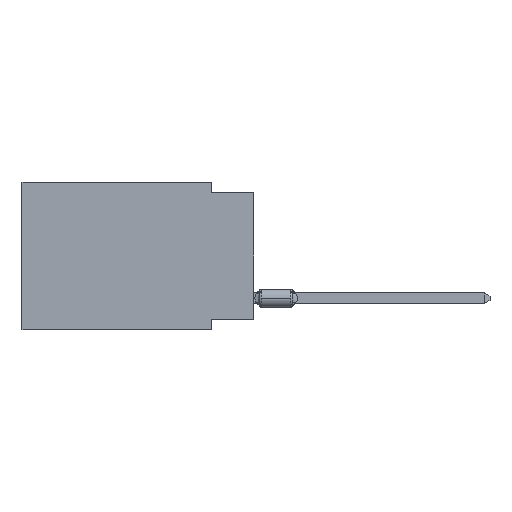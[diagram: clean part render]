
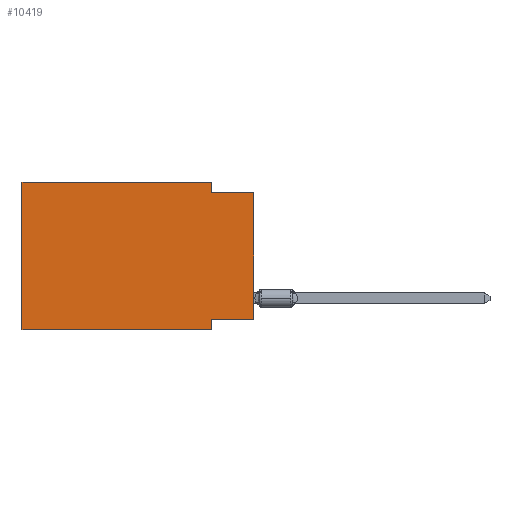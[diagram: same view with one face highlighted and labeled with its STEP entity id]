
A CAD part, left-side view. The second image highlights one B-rep face of the part: STEP entity #10419.
In plain terms, the highlighted planar face has unit normal (-1, 0, 0).
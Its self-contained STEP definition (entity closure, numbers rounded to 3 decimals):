
#98 = LINE ( 'NONE', #17383, #18273 ) ;
#118 = CARTESIAN_POINT ( 'NONE',  ( 0., 13.97, 0. ) ) ;
#355 = ORIENTED_EDGE ( 'NONE', *, *, #24967, .F. ) ;
#818 = EDGE_CURVE ( 'NONE', #24114, #4047, #17471, .T. ) ;
#2489 = DIRECTION ( 'NONE',  ( 0., 0., 1. ) ) ;
#2927 = LINE ( 'NONE', #19809, #13702 ) ;
#2941 = CARTESIAN_POINT ( 'NONE',  ( 0., 0., -8.255 ) ) ;
#3086 = DIRECTION ( 'NONE',  ( 0., -1., 0. ) ) ;
#3266 = AXIS2_PLACEMENT_3D ( 'NONE', #118, #14785, #27245 ) ;
#4047 = VERTEX_POINT ( 'NONE', #27124 ) ;
#4933 = EDGE_CURVE ( 'NONE', #27337, #19871, #8294, .T. ) ;
#5294 = CARTESIAN_POINT ( 'NONE',  ( 0., 13.97, -8.89 ) ) ;
#5333 = EDGE_CURVE ( 'NONE', #19871, #11770, #98, .T. ) ;
#5470 = VECTOR ( 'NONE', #3086, 1000. ) ;
#6380 = CARTESIAN_POINT ( 'NONE',  ( 0., 2.54, 0. ) ) ;
#6936 = CARTESIAN_POINT ( 'NONE',  ( 0., 0., -8.255 ) ) ;
#7113 = EDGE_CURVE ( 'NONE', #27337, #24316, #22320, .T. ) ;
#8066 = LINE ( 'NONE', #21229, #18975 ) ;
#8294 = LINE ( 'NONE', #16730, #24438 ) ;
#8352 = DIRECTION ( 'NONE',  ( 0., 0., 1. ) ) ;
#10286 = CARTESIAN_POINT ( 'NONE',  ( 0., 0., 0. ) ) ;
#10288 = VERTEX_POINT ( 'NONE', #22146 ) ;
#10419 = ADVANCED_FACE ( 'NONE', ( #19072 ), #16859, .F. ) ;
#10616 = ORIENTED_EDGE ( 'NONE', *, *, #5333, .F. ) ;
#10738 = ORIENTED_EDGE ( 'NONE', *, *, #4933, .F. ) ;
#11770 = VERTEX_POINT ( 'NONE', #6380 ) ;
#11837 = DIRECTION ( 'NONE',  ( 0., 0., -1. ) ) ;
#12304 = VECTOR ( 'NONE', #8352, 1000. ) ;
#12635 = LINE ( 'NONE', #10286, #12304 ) ;
#13702 = VECTOR ( 'NONE', #17733, 1000. ) ;
#13925 = CARTESIAN_POINT ( 'NONE',  ( 0., 2.54, 0. ) ) ;
#14785 = DIRECTION ( 'NONE',  ( 1., 0., 0. ) ) ;
#15174 = VERTEX_POINT ( 'NONE', #18617 ) ;
#15389 = DIRECTION ( 'NONE',  ( 0., 1., 0. ) ) ;
#15802 = VECTOR ( 'NONE', #15389, 1000. ) ;
#16543 = CARTESIAN_POINT ( 'NONE',  ( 0., 13.97, 0. ) ) ;
#16730 = CARTESIAN_POINT ( 'NONE',  ( 0., 13.97, 0. ) ) ;
#16859 = PLANE ( 'NONE',  #3266 ) ;
#17247 = ORIENTED_EDGE ( 'NONE', *, *, #27040, .T. ) ;
#17248 = DIRECTION ( 'NONE',  ( 0., -1., 0. ) ) ;
#17383 = CARTESIAN_POINT ( 'NONE',  ( 0., 13.97, 0. ) ) ;
#17471 = LINE ( 'NONE', #6936, #15802 ) ;
#17733 = DIRECTION ( 'NONE',  ( 0., -1., 0. ) ) ;
#17815 = LINE ( 'NONE', #13925, #24587 ) ;
#17876 = EDGE_CURVE ( 'NONE', #15174, #10288, #2927, .T. ) ;
#18273 = VECTOR ( 'NONE', #17248, 1000. ) ;
#18617 = CARTESIAN_POINT ( 'NONE',  ( 0., 2.54, -0.635 ) ) ;
#18688 = CARTESIAN_POINT ( 'NONE',  ( 0., 2.54, -8.89 ) ) ;
#18728 = DIRECTION ( 'NONE',  ( 0., 0., -1. ) ) ;
#18975 = VECTOR ( 'NONE', #18728, 1000. ) ;
#19072 = FACE_OUTER_BOUND ( 'NONE', #19395, .T. ) ;
#19395 = EDGE_LOOP ( 'NONE', ( #17247, #20435, #355, #10616, #10738, #20055, #25947, #27048 ) ) ;
#19809 = CARTESIAN_POINT ( 'NONE',  ( 0., 0., -0.635 ) ) ;
#19871 = VERTEX_POINT ( 'NONE', #16543 ) ;
#20055 = ORIENTED_EDGE ( 'NONE', *, *, #7113, .T. ) ;
#20332 = CARTESIAN_POINT ( 'NONE',  ( 0., 13.97, -8.89 ) ) ;
#20435 = ORIENTED_EDGE ( 'NONE', *, *, #17876, .F. ) ;
#21229 = CARTESIAN_POINT ( 'NONE',  ( 0., 2.54, -8.89 ) ) ;
#22146 = CARTESIAN_POINT ( 'NONE',  ( 0., 0., -0.635 ) ) ;
#22320 = LINE ( 'NONE', #5294, #5470 ) ;
#24114 = VERTEX_POINT ( 'NONE', #2941 ) ;
#24316 = VERTEX_POINT ( 'NONE', #18688 ) ;
#24438 = VECTOR ( 'NONE', #2489, 1000. ) ;
#24587 = VECTOR ( 'NONE', #11837, 1000. ) ;
#24967 = EDGE_CURVE ( 'NONE', #11770, #15174, #17815, .T. ) ;
#25947 = ORIENTED_EDGE ( 'NONE', *, *, #27073, .F. ) ;
#27040 = EDGE_CURVE ( 'NONE', #24114, #10288, #12635, .T. ) ;
#27048 = ORIENTED_EDGE ( 'NONE', *, *, #818, .F. ) ;
#27073 = EDGE_CURVE ( 'NONE', #4047, #24316, #8066, .T. ) ;
#27124 = CARTESIAN_POINT ( 'NONE',  ( 0., 2.54, -8.255 ) ) ;
#27245 = DIRECTION ( 'NONE',  ( 0., 0., -1. ) ) ;
#27337 = VERTEX_POINT ( 'NONE', #20332 ) ;
